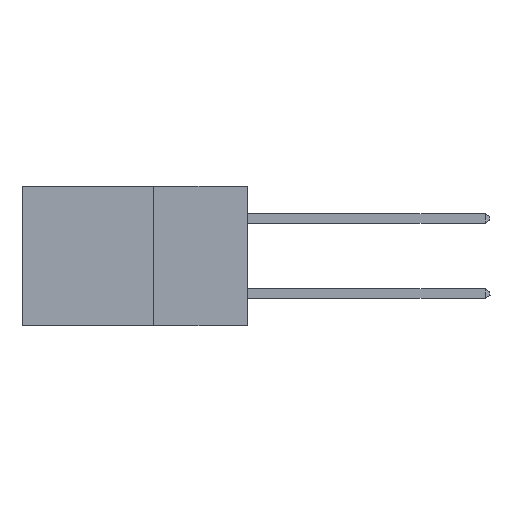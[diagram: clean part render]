
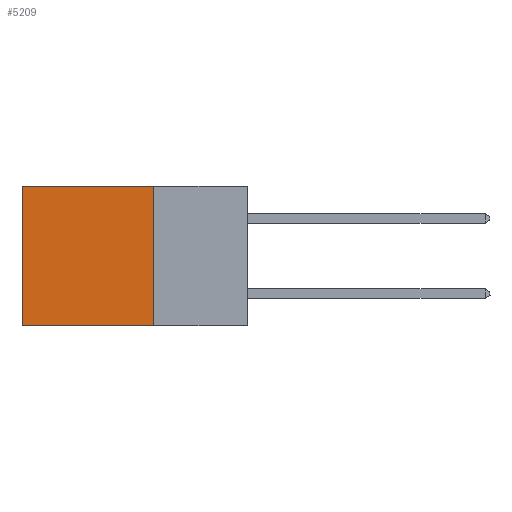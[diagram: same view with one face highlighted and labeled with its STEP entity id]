
A CAD part, left-side view. The second image highlights one B-rep face of the part: STEP entity #5209.
In plain terms, the highlighted planar face has unit normal (-1, 0, 0).
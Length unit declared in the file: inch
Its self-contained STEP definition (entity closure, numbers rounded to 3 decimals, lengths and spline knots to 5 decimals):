
#279 = EDGE_CURVE ( 'NONE', #12697, #1675, #4517, .T. ) ;
#313 = CARTESIAN_POINT ( 'NONE',  ( 0.298, 0.25, 0. ) ) ;
#1675 = VERTEX_POINT ( 'NONE', #3632 ) ;
#1781 = FACE_OUTER_BOUND ( 'NONE', #8023, .T. ) ;
#1837 = CARTESIAN_POINT ( 'NONE',  ( 0.298, 0.25, -0.37 ) ) ;
#2727 = VECTOR ( 'NONE', #7142, 39.37008 ) ;
#3000 = CARTESIAN_POINT ( 'NONE',  ( 0.298, 0.25, 0. ) ) ;
#3588 = LINE ( 'NONE', #1837, #5679 ) ;
#3632 = CARTESIAN_POINT ( 'NONE',  ( 0.298, 0.25, -0.37 ) ) ;
#3778 = LINE ( 'NONE', #11158, #6167 ) ;
#4363 = VECTOR ( 'NONE', #9017, 39.37008 ) ;
#4517 = LINE ( 'NONE', #7962, #4363 ) ;
#4814 = DIRECTION ( 'NONE',  ( 0., 1., 0. ) ) ;
#5209 = ADVANCED_FACE ( 'NONE', ( #1781 ), #12014, .F. ) ;
#5506 = CARTESIAN_POINT ( 'NONE',  ( 0.298, 0.6, -0.37 ) ) ;
#5628 = AXIS2_PLACEMENT_3D ( 'NONE', #3000, #11146, #7323 ) ;
#5679 = VECTOR ( 'NONE', #4814, 39.37008 ) ;
#5709 = EDGE_CURVE ( 'NONE', #12697, #12910, #9517, .T. ) ;
#5976 = ORIENTED_EDGE ( 'NONE', *, *, #5709, .T. ) ;
#6167 = VECTOR ( 'NONE', #6997, 39.37008 ) ;
#6374 = ORIENTED_EDGE ( 'NONE', *, *, #8072, .F. ) ;
#6596 = ORIENTED_EDGE ( 'NONE', *, *, #9470, .T. ) ;
#6997 = DIRECTION ( 'NONE',  ( 0., 0., -1. ) ) ;
#7142 = DIRECTION ( 'NONE',  ( 0., 1., 0. ) ) ;
#7213 = ORIENTED_EDGE ( 'NONE', *, *, #279, .F. ) ;
#7323 = DIRECTION ( 'NONE',  ( 0., 0., -1. ) ) ;
#7898 = CARTESIAN_POINT ( 'NONE',  ( 0.298, 0.25, 0. ) ) ;
#7962 = CARTESIAN_POINT ( 'NONE',  ( 0.298, 0.25, 0. ) ) ;
#8023 = EDGE_LOOP ( 'NONE', ( #6596, #6374, #7213, #5976 ) ) ;
#8072 = EDGE_CURVE ( 'NONE', #1675, #12475, #3588, .T. ) ;
#9017 = DIRECTION ( 'NONE',  ( 0., 0., -1. ) ) ;
#9470 = EDGE_CURVE ( 'NONE', #12910, #12475, #3778, .T. ) ;
#9517 = LINE ( 'NONE', #313, #2727 ) ;
#11146 = DIRECTION ( 'NONE',  ( 1., 0., 0. ) ) ;
#11158 = CARTESIAN_POINT ( 'NONE',  ( 0.298, 0.6, 0. ) ) ;
#11390 = CARTESIAN_POINT ( 'NONE',  ( 0.298, 0.6, 0. ) ) ;
#12014 = PLANE ( 'NONE',  #5628 ) ;
#12475 = VERTEX_POINT ( 'NONE', #5506 ) ;
#12697 = VERTEX_POINT ( 'NONE', #7898 ) ;
#12910 = VERTEX_POINT ( 'NONE', #11390 ) ;
